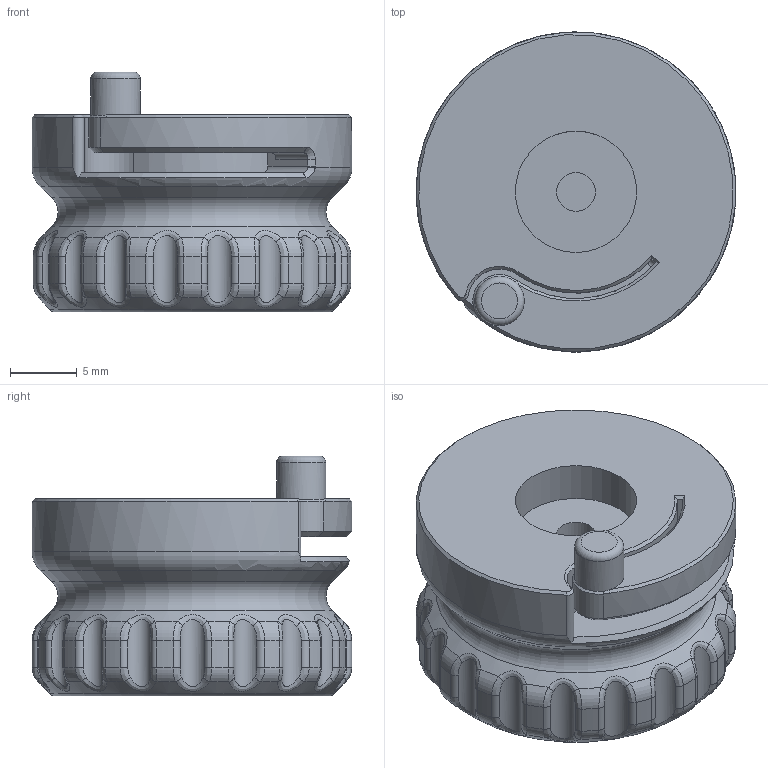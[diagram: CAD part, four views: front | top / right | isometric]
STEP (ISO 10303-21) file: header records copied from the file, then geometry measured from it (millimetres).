
FILE_DESCRIPTION(/* description */ (''),/* implementation_level */ '2;1');
FILE_NAME(/* name */ 'Cartridge Release Knob.step',/* time_stamp */ '2021-05-10T17:22:09-04:00',/* author */ (''),/* organization */ (''),/* preprocessor_version */ 'ST-DEVELOPER v18.1',/* originating_system */ 'Autodesk Translation Framework v10.6.0.1341',/* authorisation */ '');
FILE_SCHEMA (('AUTOMOTIVE_DESIGN { 1 0 10303 214 3 1 1 }'));
Length unit declared in the file: millimetre
Products named in the file (1): 3FTech Logo Cartridge Release Knob
Bounding box: 24 x 24 x 18 mm (x, y, z)
Volume: 5593.2 mm3; surface area: 2492.7 mm2
Topology: 1 solids, 1 shells, 297 faces, 693 edges, 398 vertices
Faces by surface type: bspline 124, cylinder 97, torus 47, cone 15, plane 14
Full cylindrical faces by diameter (mm): 2.9 x1, 3.7 x1, 9.1 x1, 16.6 x1, 18.6 x1
Entity records: 12524 total; most frequent: CARTESIAN_POINT 6453, ORIENTED_EDGE 1374, DIRECTION 1084, EDGE_CURVE 687, AXIS2_PLACEMENT_3D 478, VERTEX_POINT 398, CIRCLE 304, EDGE_LOOP 303
